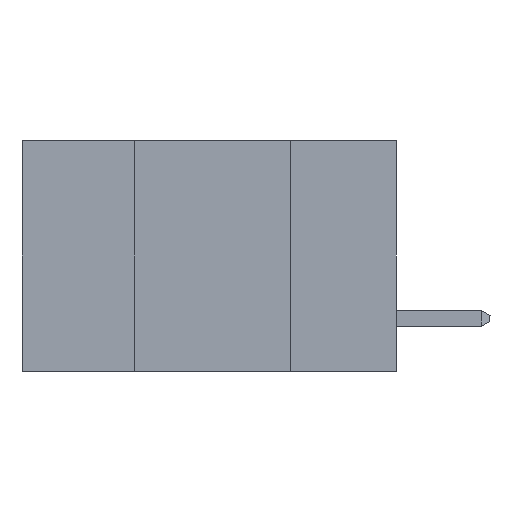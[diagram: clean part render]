
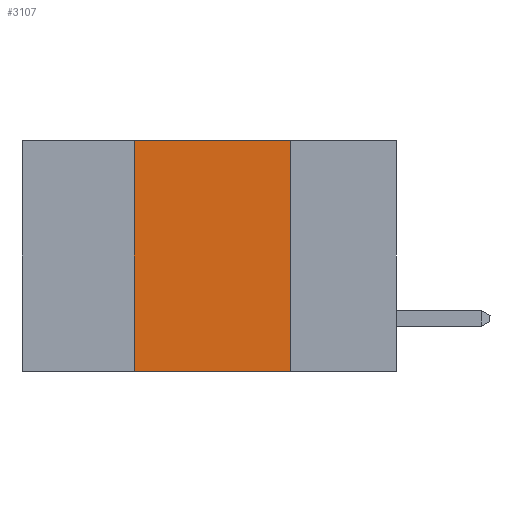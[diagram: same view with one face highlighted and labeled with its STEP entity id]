
A CAD part, left-side view. The second image highlights one B-rep face of the part: STEP entity #3107.
In plain terms, the highlighted planar face has unit normal (-1, 0, 0).
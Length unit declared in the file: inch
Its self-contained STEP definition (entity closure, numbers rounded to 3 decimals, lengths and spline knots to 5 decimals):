
#221 = EDGE_CURVE ( 'NONE', #6910, #9083, #8524, .T. ) ;
#385 = CARTESIAN_POINT ( 'NONE',  ( 0., 0.6, -0.37 ) ) ;
#610 = ORIENTED_EDGE ( 'NONE', *, *, #221, .F. ) ;
#1066 = DIRECTION ( 'NONE',  ( 1., 0., 0. ) ) ;
#1069 = DIRECTION ( 'NONE',  ( 0., -1., 0. ) ) ;
#1267 = ORIENTED_EDGE ( 'NONE', *, *, #1912, .F. ) ;
#1316 = ORIENTED_EDGE ( 'NONE', *, *, #5006, .F. ) ;
#1912 = EDGE_CURVE ( 'NONE', #1958, #6910, #2368, .T. ) ;
#1958 = VERTEX_POINT ( 'NONE', #11267 ) ;
#2078 = DIRECTION ( 'NONE',  ( 0., 0., 1. ) ) ;
#2120 = CARTESIAN_POINT ( 'NONE',  ( 0., 0.6, 0. ) ) ;
#2368 = LINE ( 'NONE', #6755, #12152 ) ;
#2576 = CARTESIAN_POINT ( 'NONE',  ( 0., 0.17, -0.37 ) ) ;
#3107 = ADVANCED_FACE ( 'NONE', ( #5325 ), #8680, .F. ) ;
#3440 = EDGE_LOOP ( 'NONE', ( #1316, #610, #1267, #7603 ) ) ;
#4225 = CARTESIAN_POINT ( 'NONE',  ( 0., 0.42, 0. ) ) ;
#4244 = VERTEX_POINT ( 'NONE', #2576 ) ;
#5006 = EDGE_CURVE ( 'NONE', #9083, #4244, #9003, .T. ) ;
#5325 = FACE_OUTER_BOUND ( 'NONE', #3440, .T. ) ;
#5494 = EDGE_CURVE ( 'NONE', #1958, #4244, #10812, .T. ) ;
#6131 = VECTOR ( 'NONE', #1069, 39.37008 ) ;
#6752 = CARTESIAN_POINT ( 'NONE',  ( 0., 0.6, 0. ) ) ;
#6755 = CARTESIAN_POINT ( 'NONE',  ( 0., 0.42, 0. ) ) ;
#6910 = VERTEX_POINT ( 'NONE', #4225 ) ;
#7473 = DIRECTION ( 'NONE',  ( 0., 0., -1. ) ) ;
#7603 = ORIENTED_EDGE ( 'NONE', *, *, #5494, .T. ) ;
#8524 = LINE ( 'NONE', #6752, #6131 ) ;
#8680 = PLANE ( 'NONE',  #12214 ) ;
#8819 = DIRECTION ( 'NONE',  ( 0., 0., -1. ) ) ;
#9001 = CARTESIAN_POINT ( 'NONE',  ( 0., 0.17, 0. ) ) ;
#9003 = LINE ( 'NONE', #10301, #11366 ) ;
#9083 = VERTEX_POINT ( 'NONE', #9001 ) ;
#9477 = VECTOR ( 'NONE', #11766, 39.37008 ) ;
#10301 = CARTESIAN_POINT ( 'NONE',  ( 0., 0.17, 0. ) ) ;
#10812 = LINE ( 'NONE', #385, #9477 ) ;
#11267 = CARTESIAN_POINT ( 'NONE',  ( 0., 0.42, -0.37 ) ) ;
#11366 = VECTOR ( 'NONE', #7473, 39.37008 ) ;
#11766 = DIRECTION ( 'NONE',  ( 0., -1., 0. ) ) ;
#12152 = VECTOR ( 'NONE', #2078, 39.37008 ) ;
#12214 = AXIS2_PLACEMENT_3D ( 'NONE', #2120, #1066, #8819 ) ;
